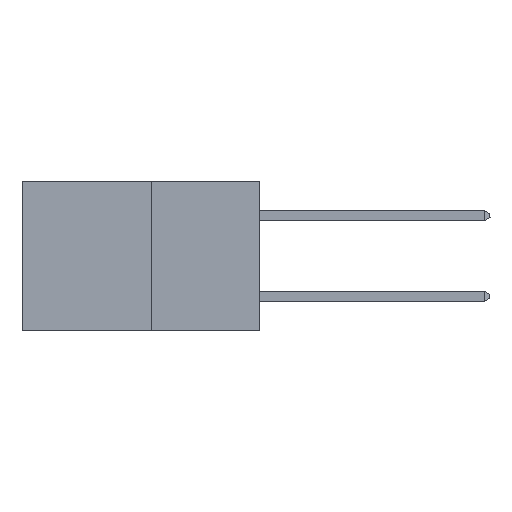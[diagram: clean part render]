
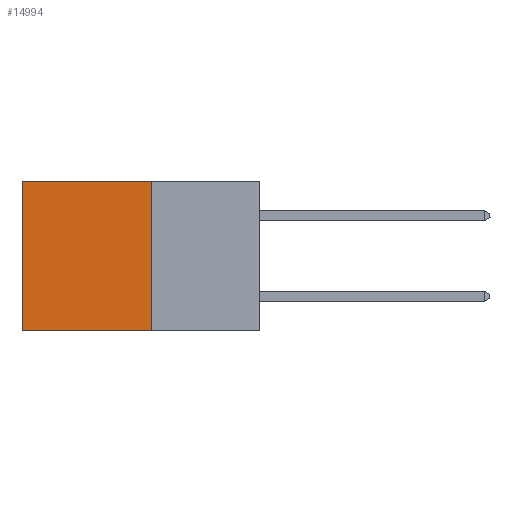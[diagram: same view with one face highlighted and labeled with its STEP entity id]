
A CAD part, left-side view. The second image highlights one B-rep face of the part: STEP entity #14994.
In plain terms, the highlighted planar face has unit normal (-1, 0, 0).
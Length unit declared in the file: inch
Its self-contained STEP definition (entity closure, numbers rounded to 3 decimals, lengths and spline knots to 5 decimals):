
#535 = VECTOR ( 'NONE', #2884, 39.37008 ) ;
#1588 = PLANE ( 'NONE',  #8885 ) ;
#2161 = EDGE_LOOP ( 'NONE', ( #6993, #7885, #14009, #4840 ) ) ;
#2268 = DIRECTION ( 'NONE',  ( 0., 1., 0. ) ) ;
#2884 = DIRECTION ( 'NONE',  ( 0., 0., -1. ) ) ;
#3065 = CARTESIAN_POINT ( 'NONE',  ( 0.277, 0.59, 0. ) ) ;
#3225 = CARTESIAN_POINT ( 'NONE',  ( 0.277, 0.59, -0.37 ) ) ;
#3366 = VECTOR ( 'NONE', #7009, 39.37008 ) ;
#3972 = DIRECTION ( 'NONE',  ( 0., 0., -1. ) ) ;
#4680 = CARTESIAN_POINT ( 'NONE',  ( 0.277, 0.27, 0. ) ) ;
#4771 = VERTEX_POINT ( 'NONE', #3065 ) ;
#4840 = ORIENTED_EDGE ( 'NONE', *, *, #11851, .T. ) ;
#5146 = VERTEX_POINT ( 'NONE', #4680 ) ;
#5328 = CARTESIAN_POINT ( 'NONE',  ( 0.277, 0.27, -0.37 ) ) ;
#5763 = CARTESIAN_POINT ( 'NONE',  ( 0.277, 0.59, -0.37 ) ) ;
#6858 = LINE ( 'NONE', #5763, #13157 ) ;
#6907 = VERTEX_POINT ( 'NONE', #3225 ) ;
#6993 = ORIENTED_EDGE ( 'NONE', *, *, #7638, .T. ) ;
#7009 = DIRECTION ( 'NONE',  ( 0., 1., 0. ) ) ;
#7638 = EDGE_CURVE ( 'NONE', #4771, #6907, #6858, .T. ) ;
#7885 = ORIENTED_EDGE ( 'NONE', *, *, #9130, .F. ) ;
#8067 = EDGE_CURVE ( 'NONE', #5146, #8511, #9977, .T. ) ;
#8511 = VERTEX_POINT ( 'NONE', #11914 ) ;
#8671 = VECTOR ( 'NONE', #2268, 39.37008 ) ;
#8885 = AXIS2_PLACEMENT_3D ( 'NONE', #9862, #11068, #3972 ) ;
#9130 = EDGE_CURVE ( 'NONE', #8511, #6907, #14916, .T. ) ;
#9340 = CARTESIAN_POINT ( 'NONE',  ( 0.277, 0.27, 0. ) ) ;
#9862 = CARTESIAN_POINT ( 'NONE',  ( 0.277, 0.27, -0.37 ) ) ;
#9907 = FACE_OUTER_BOUND ( 'NONE', #2161, .T. ) ;
#9977 = LINE ( 'NONE', #5328, #535 ) ;
#11068 = DIRECTION ( 'NONE',  ( 1., 0., 0. ) ) ;
#11729 = CARTESIAN_POINT ( 'NONE',  ( 0.277, 0.27, -0.37 ) ) ;
#11851 = EDGE_CURVE ( 'NONE', #5146, #4771, #12807, .T. ) ;
#11914 = CARTESIAN_POINT ( 'NONE',  ( 0.277, 0.27, -0.37 ) ) ;
#12807 = LINE ( 'NONE', #9340, #3366 ) ;
#13157 = VECTOR ( 'NONE', #13978, 39.37008 ) ;
#13978 = DIRECTION ( 'NONE',  ( 0., 0., -1. ) ) ;
#14009 = ORIENTED_EDGE ( 'NONE', *, *, #8067, .F. ) ;
#14916 = LINE ( 'NONE', #11729, #8671 ) ;
#14994 = ADVANCED_FACE ( 'NONE', ( #9907 ), #1588, .F. ) ;
